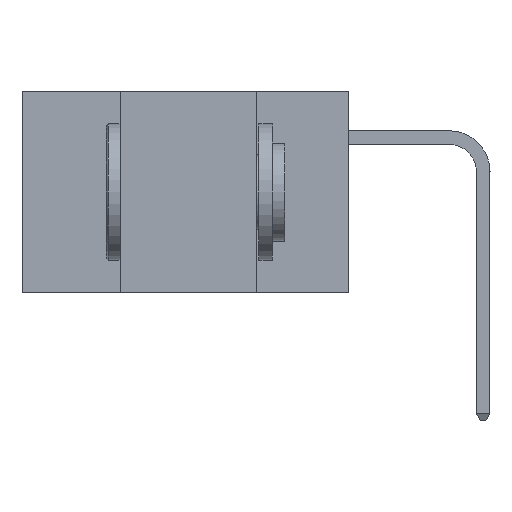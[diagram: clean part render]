
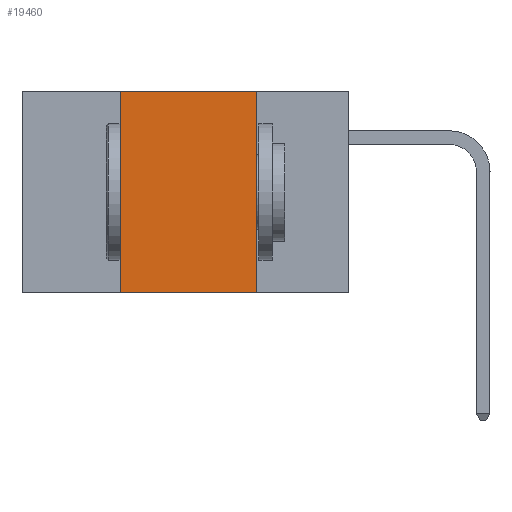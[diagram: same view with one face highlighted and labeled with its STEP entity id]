
A CAD part, left-side view. The second image highlights one B-rep face of the part: STEP entity #19460.
In plain terms, the highlighted planar face has unit normal (-1, 0, 0).
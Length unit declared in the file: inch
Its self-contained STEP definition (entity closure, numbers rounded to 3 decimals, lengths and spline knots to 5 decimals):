
#130 = DIRECTION ( 'NONE',  ( 0., -1., 0. ) ) ;
#1976 = DIRECTION ( 'NONE',  ( 0., 0., 1. ) ) ;
#2093 = CARTESIAN_POINT ( 'NONE',  ( 0., 0.6, 0. ) ) ;
#2151 = DIRECTION ( 'NONE',  ( 1., 0., 0. ) ) ;
#2578 = LINE ( 'NONE', #2093, #22570 ) ;
#2803 = EDGE_CURVE ( 'NONE', #7419, #12796, #2578, .T. ) ;
#3611 = FACE_OUTER_BOUND ( 'NONE', #21040, .T. ) ;
#4865 = VECTOR ( 'NONE', #1976, 39.37008 ) ;
#6961 = VERTEX_POINT ( 'NONE', #12109 ) ;
#7370 = ORIENTED_EDGE ( 'NONE', *, *, #15007, .F. ) ;
#7419 = VERTEX_POINT ( 'NONE', #17201 ) ;
#7511 = VERTEX_POINT ( 'NONE', #12087 ) ;
#8808 = VECTOR ( 'NONE', #20083, 39.37008 ) ;
#9421 = LINE ( 'NONE', #18173, #8808 ) ;
#10527 = ORIENTED_EDGE ( 'NONE', *, *, #19412, .F. ) ;
#10632 = EDGE_CURVE ( 'NONE', #6961, #7511, #16025, .T. ) ;
#12087 = CARTESIAN_POINT ( 'NONE',  ( 0., 0.17, -0.37 ) ) ;
#12109 = CARTESIAN_POINT ( 'NONE',  ( 0., 0.42, -0.37 ) ) ;
#12796 = VERTEX_POINT ( 'NONE', #14833 ) ;
#13871 = CARTESIAN_POINT ( 'NONE',  ( 0., 0.6, 0. ) ) ;
#14012 = ORIENTED_EDGE ( 'NONE', *, *, #10632, .T. ) ;
#14833 = CARTESIAN_POINT ( 'NONE',  ( 0., 0.17, 0. ) ) ;
#15007 = EDGE_CURVE ( 'NONE', #12796, #7511, #9421, .T. ) ;
#15218 = LINE ( 'NONE', #15628, #4865 ) ;
#15628 = CARTESIAN_POINT ( 'NONE',  ( 0., 0.42, 0. ) ) ;
#15800 = DIRECTION ( 'NONE',  ( 0., 0., -1. ) ) ;
#16025 = LINE ( 'NONE', #22305, #21105 ) ;
#16277 = AXIS2_PLACEMENT_3D ( 'NONE', #13871, #2151, #15800 ) ;
#16451 = ORIENTED_EDGE ( 'NONE', *, *, #2803, .F. ) ;
#17201 = CARTESIAN_POINT ( 'NONE',  ( 0., 0.42, 0. ) ) ;
#18173 = CARTESIAN_POINT ( 'NONE',  ( 0., 0.17, 0. ) ) ;
#19412 = EDGE_CURVE ( 'NONE', #6961, #7419, #15218, .T. ) ;
#19460 = ADVANCED_FACE ( 'NONE', ( #3611 ), #21462, .F. ) ;
#20083 = DIRECTION ( 'NONE',  ( 0., 0., -1. ) ) ;
#20383 = DIRECTION ( 'NONE',  ( 0., -1., 0. ) ) ;
#21040 = EDGE_LOOP ( 'NONE', ( #7370, #16451, #10527, #14012 ) ) ;
#21105 = VECTOR ( 'NONE', #20383, 39.37008 ) ;
#21462 = PLANE ( 'NONE',  #16277 ) ;
#22305 = CARTESIAN_POINT ( 'NONE',  ( 0., 0.6, -0.37 ) ) ;
#22570 = VECTOR ( 'NONE', #130, 39.37008 ) ;
